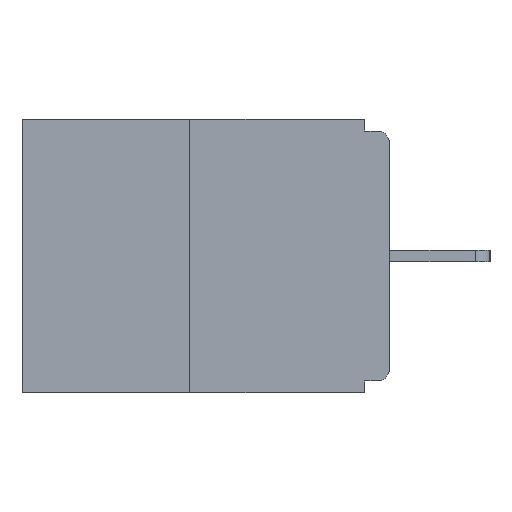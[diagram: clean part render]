
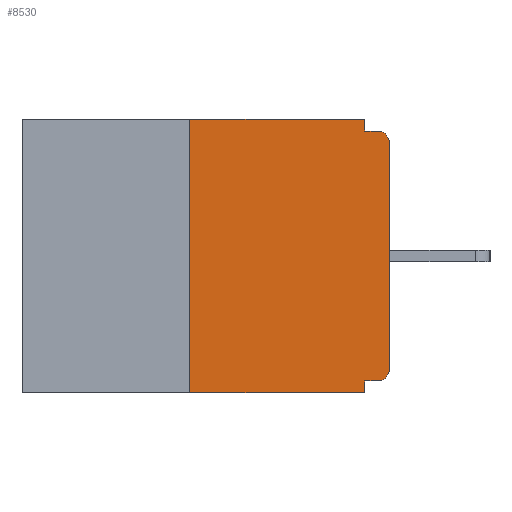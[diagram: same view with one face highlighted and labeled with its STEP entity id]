
A CAD part, left-side view. The second image highlights one B-rep face of the part: STEP entity #8530.
In plain terms, the highlighted planar face has unit normal (-1, 0, 0).
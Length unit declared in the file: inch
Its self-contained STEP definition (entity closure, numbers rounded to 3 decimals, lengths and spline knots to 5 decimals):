
#45 = EDGE_CURVE ( 'NONE', #14676, #5255, #8415, .T. ) ;
#703 = CARTESIAN_POINT ( 'NONE',  ( 0., 0.031, -0.343 ) ) ;
#892 = DIRECTION ( 'NONE',  ( 1., 0., 0. ) ) ;
#939 = EDGE_CURVE ( 'NONE', #25184, #25864, #15696, .T. ) ;
#1111 = ORIENTED_EDGE ( 'NONE', *, *, #24301, .T. ) ;
#1183 = LINE ( 'NONE', #2401, #16539 ) ;
#1289 = CARTESIAN_POINT ( 'NONE',  ( 0., 0.015, -0.313 ) ) ;
#1336 = ORIENTED_EDGE ( 'NONE', *, *, #16268, .F. ) ;
#1428 = EDGE_CURVE ( 'NONE', #5255, #4268, #3817, .T. ) ;
#1899 = CIRCLE ( 'NONE', #4205, 0.015 ) ;
#1931 = CARTESIAN_POINT ( 'NONE',  ( 0., 0.015, -0.03 ) ) ;
#2050 = DIRECTION ( 'NONE',  ( 0., -1., 0. ) ) ;
#2401 = CARTESIAN_POINT ( 'NONE',  ( 0., 0., -0.015 ) ) ;
#2848 = CARTESIAN_POINT ( 'NONE',  ( 0., 0.25, -0.343 ) ) ;
#3233 = DIRECTION ( 'NONE',  ( 0., -1., 0. ) ) ;
#3395 = DIRECTION ( 'NONE',  ( 0., 0., -1. ) ) ;
#3817 = LINE ( 'NONE', #25191, #8483 ) ;
#4205 = AXIS2_PLACEMENT_3D ( 'NONE', #1931, #24252, #10208 ) ;
#4268 = VERTEX_POINT ( 'NONE', #10312 ) ;
#4443 = VECTOR ( 'NONE', #3233, 39.37008 ) ;
#4543 = DIRECTION ( 'NONE',  ( 0., 1., 0. ) ) ;
#5224 = ORIENTED_EDGE ( 'NONE', *, *, #939, .T. ) ;
#5255 = VERTEX_POINT ( 'NONE', #5808 ) ;
#5289 = VECTOR ( 'NONE', #17154, 39.37008 ) ;
#5393 = DIRECTION ( 'NONE',  ( 0., 0., -1. ) ) ;
#5808 = CARTESIAN_POINT ( 'NONE',  ( 0., 0.031, 0. ) ) ;
#6074 = CARTESIAN_POINT ( 'NONE',  ( 0., 0.25, 0. ) ) ;
#6509 = LINE ( 'NONE', #16520, #13365 ) ;
#6653 = CARTESIAN_POINT ( 'NONE',  ( 0., 0.031, -0.328 ) ) ;
#7287 = PLANE ( 'NONE',  #12044 ) ;
#7581 = CARTESIAN_POINT ( 'NONE',  ( 0., 0.031, -0.343 ) ) ;
#8237 = DIRECTION ( 'NONE',  ( 0., 0., 1. ) ) ;
#8238 = EDGE_LOOP ( 'NONE', ( #10060, #11340, #5224, #24916, #8467, #1111, #11024, #12706, #1336, #15575 ) ) ;
#8415 = LINE ( 'NONE', #9030, #5289 ) ;
#8467 = ORIENTED_EDGE ( 'NONE', *, *, #16129, .F. ) ;
#8483 = VECTOR ( 'NONE', #3395, 39.37008 ) ;
#8530 = ADVANCED_FACE ( 'NONE', ( #13961 ), #7287, .F. ) ;
#8726 = VERTEX_POINT ( 'NONE', #13644 ) ;
#8738 = DIRECTION ( 'NONE',  ( 0., 0., 1. ) ) ;
#8808 = EDGE_CURVE ( 'NONE', #25184, #14676, #11101, .T. ) ;
#9028 = VERTEX_POINT ( 'NONE', #11769 ) ;
#9030 = CARTESIAN_POINT ( 'NONE',  ( 0., 0.46, 0. ) ) ;
#9264 = DIRECTION ( 'NONE',  ( 0., 0., -1. ) ) ;
#9973 = VERTEX_POINT ( 'NONE', #6653 ) ;
#10060 = ORIENTED_EDGE ( 'NONE', *, *, #45, .F. ) ;
#10208 = DIRECTION ( 'NONE',  ( 0., 0., -1. ) ) ;
#10312 = CARTESIAN_POINT ( 'NONE',  ( 0., 0.031, -0.015 ) ) ;
#10922 = EDGE_CURVE ( 'NONE', #18168, #9028, #1899, .T. ) ;
#11024 = ORIENTED_EDGE ( 'NONE', *, *, #24257, .T. ) ;
#11101 = LINE ( 'NONE', #6074, #17369 ) ;
#11340 = ORIENTED_EDGE ( 'NONE', *, *, #8808, .F. ) ;
#11769 = CARTESIAN_POINT ( 'NONE',  ( 0., 0.015, -0.015 ) ) ;
#12044 = AXIS2_PLACEMENT_3D ( 'NONE', #23203, #892, #9264 ) ;
#12645 = LINE ( 'NONE', #16955, #15156 ) ;
#12706 = ORIENTED_EDGE ( 'NONE', *, *, #10922, .T. ) ;
#12760 = CARTESIAN_POINT ( 'NONE',  ( 0., 0.015, -0.328 ) ) ;
#13365 = VECTOR ( 'NONE', #4543, 39.37008 ) ;
#13644 = CARTESIAN_POINT ( 'NONE',  ( 0., 0., -0.313 ) ) ;
#13961 = FACE_OUTER_BOUND ( 'NONE', #8238, .T. ) ;
#14676 = VERTEX_POINT ( 'NONE', #24412 ) ;
#15156 = VECTOR ( 'NONE', #8738, 39.37008 ) ;
#15302 = DIRECTION ( 'NONE',  ( -1., 0., 0. ) ) ;
#15575 = ORIENTED_EDGE ( 'NONE', *, *, #1428, .F. ) ;
#15696 = LINE ( 'NONE', #19081, #4443 ) ;
#16129 = EDGE_CURVE ( 'NONE', #19064, #9973, #6509, .T. ) ;
#16268 = EDGE_CURVE ( 'NONE', #4268, #9028, #1183, .T. ) ;
#16520 = CARTESIAN_POINT ( 'NONE',  ( 0., 0., -0.328 ) ) ;
#16539 = VECTOR ( 'NONE', #2050, 39.37008 ) ;
#16955 = CARTESIAN_POINT ( 'NONE',  ( 0., 0., 0. ) ) ;
#17154 = DIRECTION ( 'NONE',  ( 0., -1., 0. ) ) ;
#17369 = VECTOR ( 'NONE', #8237, 39.37008 ) ;
#17687 = VECTOR ( 'NONE', #5393, 39.37008 ) ;
#18168 = VERTEX_POINT ( 'NONE', #23232 ) ;
#18471 = AXIS2_PLACEMENT_3D ( 'NONE', #1289, #15302, #25305 ) ;
#19064 = VERTEX_POINT ( 'NONE', #12760 ) ;
#19081 = CARTESIAN_POINT ( 'NONE',  ( 0., 0.46, -0.343 ) ) ;
#20308 = EDGE_CURVE ( 'NONE', #9973, #25864, #21429, .T. ) ;
#21429 = LINE ( 'NONE', #7581, #17687 ) ;
#22009 = CIRCLE ( 'NONE', #18471, 0.015 ) ;
#23203 = CARTESIAN_POINT ( 'NONE',  ( 0., 0.46, 0. ) ) ;
#23232 = CARTESIAN_POINT ( 'NONE',  ( 0., 0., -0.03 ) ) ;
#24252 = DIRECTION ( 'NONE',  ( -1., 0., 0. ) ) ;
#24257 = EDGE_CURVE ( 'NONE', #8726, #18168, #12645, .T. ) ;
#24301 = EDGE_CURVE ( 'NONE', #19064, #8726, #22009, .T. ) ;
#24412 = CARTESIAN_POINT ( 'NONE',  ( 0., 0.25, 0. ) ) ;
#24916 = ORIENTED_EDGE ( 'NONE', *, *, #20308, .F. ) ;
#25184 = VERTEX_POINT ( 'NONE', #2848 ) ;
#25191 = CARTESIAN_POINT ( 'NONE',  ( 0., 0.031, 0. ) ) ;
#25305 = DIRECTION ( 'NONE',  ( 0., 0., -1. ) ) ;
#25864 = VERTEX_POINT ( 'NONE', #703 ) ;
